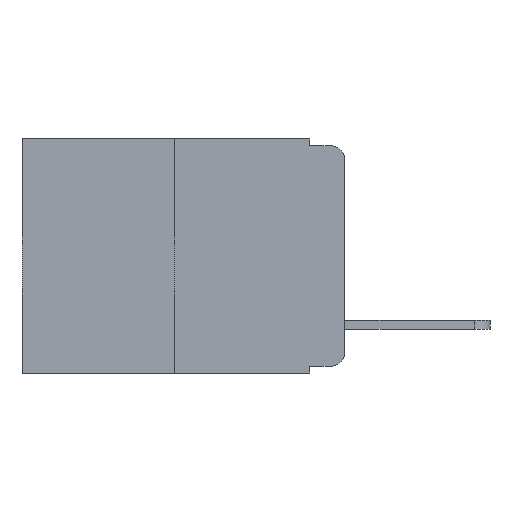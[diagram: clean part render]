
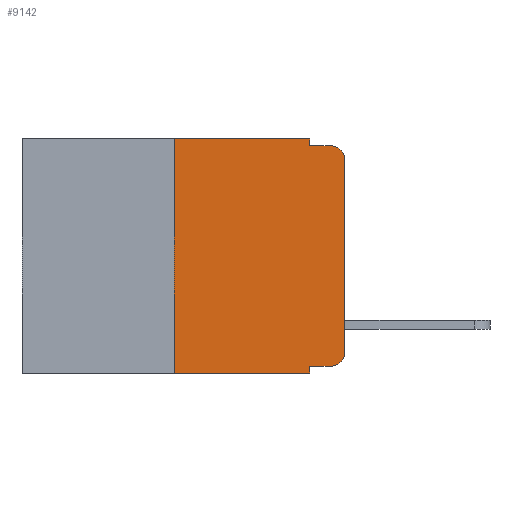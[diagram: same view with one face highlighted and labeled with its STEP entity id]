
A CAD part, left-side view. The second image highlights one B-rep face of the part: STEP entity #9142.
In plain terms, the highlighted planar face has unit normal (-1, 0, 0).
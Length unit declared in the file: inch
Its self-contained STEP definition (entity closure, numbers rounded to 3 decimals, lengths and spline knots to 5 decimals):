
#240 = DIRECTION ( 'NONE',  ( 0., 0., -1. ) ) ;
#306 = DIRECTION ( 'NONE',  ( -1., 0., 0. ) ) ;
#309 = CARTESIAN_POINT ( 'NONE',  ( 0., 0.02, -0.03 ) ) ;
#319 = DIRECTION ( 'NONE',  ( 0., 0., -1. ) ) ;
#512 = LINE ( 'NONE', #15917, #18431 ) ;
#799 = CARTESIAN_POINT ( 'NONE',  ( 0., 0.051, -0.01 ) ) ;
#902 = ORIENTED_EDGE ( 'NONE', *, *, #2876, .T. ) ;
#930 = VERTEX_POINT ( 'NONE', #17466 ) ;
#1141 = LINE ( 'NONE', #6613, #17046 ) ;
#1346 = CARTESIAN_POINT ( 'NONE',  ( 0., 0.051, 0. ) ) ;
#1368 = VERTEX_POINT ( 'NONE', #15090 ) ;
#1692 = VERTEX_POINT ( 'NONE', #10753 ) ;
#1945 = CARTESIAN_POINT ( 'NONE',  ( 0., 0.051, -0.01 ) ) ;
#2090 = DIRECTION ( 'NONE',  ( -1., 0., 0. ) ) ;
#2108 = DIRECTION ( 'NONE',  ( 0., 0., -1. ) ) ;
#2209 = ORIENTED_EDGE ( 'NONE', *, *, #18129, .F. ) ;
#2416 = ORIENTED_EDGE ( 'NONE', *, *, #13128, .T. ) ;
#2447 = DIRECTION ( 'NONE',  ( 0., -1., 0. ) ) ;
#2486 = VECTOR ( 'NONE', #11408, 39.37008 ) ;
#2672 = LINE ( 'NONE', #3365, #14800 ) ;
#2876 = EDGE_CURVE ( 'NONE', #14019, #7792, #11787, .T. ) ;
#3004 = DIRECTION ( 'NONE',  ( 0., 0., -1. ) ) ;
#3306 = DIRECTION ( 'NONE',  ( 0., -1., 0. ) ) ;
#3309 = CARTESIAN_POINT ( 'NONE',  ( 0., 0., -0.313 ) ) ;
#3356 = EDGE_CURVE ( 'NONE', #7792, #16641, #16791, .T. ) ;
#3365 = CARTESIAN_POINT ( 'NONE',  ( 0., 0.473, -0.343 ) ) ;
#3799 = ORIENTED_EDGE ( 'NONE', *, *, #18676, .F. ) ;
#4117 = ORIENTED_EDGE ( 'NONE', *, *, #11652, .T. ) ;
#4734 = CARTESIAN_POINT ( 'NONE',  ( 0., 0., -0.03 ) ) ;
#4795 = VECTOR ( 'NONE', #17731, 39.37008 ) ;
#5307 = VERTEX_POINT ( 'NONE', #7434 ) ;
#5518 = VERTEX_POINT ( 'NONE', #16827 ) ;
#5673 = DIRECTION ( 'NONE',  ( 0., -1., 0. ) ) ;
#5927 = EDGE_CURVE ( 'NONE', #5307, #930, #1141, .T. ) ;
#6182 = CARTESIAN_POINT ( 'NONE',  ( 0., 0.473, 0. ) ) ;
#6418 = DIRECTION ( 'NONE',  ( 0., 0., 1. ) ) ;
#6613 = CARTESIAN_POINT ( 'NONE',  ( 0., 0.25, 0. ) ) ;
#6937 = LINE ( 'NONE', #11812, #2486 ) ;
#7360 = EDGE_LOOP ( 'NONE', ( #12269, #2416, #3799, #13028, #11383, #13720, #4117, #2209, #12805, #902 ) ) ;
#7434 = CARTESIAN_POINT ( 'NONE',  ( 0., 0.25, -0.343 ) ) ;
#7792 = VERTEX_POINT ( 'NONE', #3309 ) ;
#8735 = FACE_OUTER_BOUND ( 'NONE', #7360, .T. ) ;
#9129 = LINE ( 'NONE', #6182, #10120 ) ;
#9142 = ADVANCED_FACE ( 'NONE', ( #8735 ), #15395, .F. ) ;
#9941 = CIRCLE ( 'NONE', #16968, 0.02 ) ;
#10074 = VERTEX_POINT ( 'NONE', #1945 ) ;
#10120 = VECTOR ( 'NONE', #5673, 39.37008 ) ;
#10753 = CARTESIAN_POINT ( 'NONE',  ( 0., 0.051, 0. ) ) ;
#10926 = CARTESIAN_POINT ( 'NONE',  ( 0., 0., 0. ) ) ;
#11383 = ORIENTED_EDGE ( 'NONE', *, *, #11601, .F. ) ;
#11408 = DIRECTION ( 'NONE',  ( 0., -1., 0. ) ) ;
#11601 = EDGE_CURVE ( 'NONE', #930, #1692, #9129, .T. ) ;
#11652 = EDGE_CURVE ( 'NONE', #5307, #13873, #2672, .T. ) ;
#11787 = CIRCLE ( 'NONE', #19164, 0.02 ) ;
#11812 = CARTESIAN_POINT ( 'NONE',  ( 0., 0.051, -0.333 ) ) ;
#12045 = VECTOR ( 'NONE', #3004, 39.37008 ) ;
#12269 = ORIENTED_EDGE ( 'NONE', *, *, #3356, .T. ) ;
#12586 = EDGE_CURVE ( 'NONE', #1368, #14019, #6937, .T. ) ;
#12805 = ORIENTED_EDGE ( 'NONE', *, *, #12586, .T. ) ;
#13028 = ORIENTED_EDGE ( 'NONE', *, *, #15131, .F. ) ;
#13128 = EDGE_CURVE ( 'NONE', #16641, #5518, #9941, .T. ) ;
#13720 = ORIENTED_EDGE ( 'NONE', *, *, #5927, .F. ) ;
#13865 = CARTESIAN_POINT ( 'NONE',  ( 0., 0.02, -0.313 ) ) ;
#13873 = VERTEX_POINT ( 'NONE', #17879 ) ;
#14019 = VERTEX_POINT ( 'NONE', #15390 ) ;
#14800 = VECTOR ( 'NONE', #3306, 39.37008 ) ;
#14801 = VECTOR ( 'NONE', #2447, 39.37008 ) ;
#15090 = CARTESIAN_POINT ( 'NONE',  ( 0., 0.051, -0.333 ) ) ;
#15131 = EDGE_CURVE ( 'NONE', #1692, #10074, #19318, .T. ) ;
#15264 = DIRECTION ( 'NONE',  ( 0., 0., -1. ) ) ;
#15304 = DIRECTION ( 'NONE',  ( 1., 0., 0. ) ) ;
#15390 = CARTESIAN_POINT ( 'NONE',  ( 0., 0.02, -0.333 ) ) ;
#15395 = PLANE ( 'NONE',  #16258 ) ;
#15399 = CARTESIAN_POINT ( 'NONE',  ( 0., 0.473, 0. ) ) ;
#15917 = CARTESIAN_POINT ( 'NONE',  ( 0., 0.051, 0. ) ) ;
#16258 = AXIS2_PLACEMENT_3D ( 'NONE', #15399, #15304, #15264 ) ;
#16641 = VERTEX_POINT ( 'NONE', #4734 ) ;
#16791 = LINE ( 'NONE', #10926, #4795 ) ;
#16827 = CARTESIAN_POINT ( 'NONE',  ( 0., 0.02, -0.01 ) ) ;
#16968 = AXIS2_PLACEMENT_3D ( 'NONE', #309, #306, #240 ) ;
#17046 = VECTOR ( 'NONE', #6418, 39.37008 ) ;
#17466 = CARTESIAN_POINT ( 'NONE',  ( 0., 0.25, 0. ) ) ;
#17731 = DIRECTION ( 'NONE',  ( 0., 0., 1. ) ) ;
#17879 = CARTESIAN_POINT ( 'NONE',  ( 0., 0.051, -0.343 ) ) ;
#18129 = EDGE_CURVE ( 'NONE', #1368, #13873, #512, .T. ) ;
#18431 = VECTOR ( 'NONE', #319, 39.37008 ) ;
#18676 = EDGE_CURVE ( 'NONE', #10074, #5518, #18732, .T. ) ;
#18732 = LINE ( 'NONE', #799, #14801 ) ;
#19164 = AXIS2_PLACEMENT_3D ( 'NONE', #13865, #2090, #2108 ) ;
#19318 = LINE ( 'NONE', #1346, #12045 ) ;
